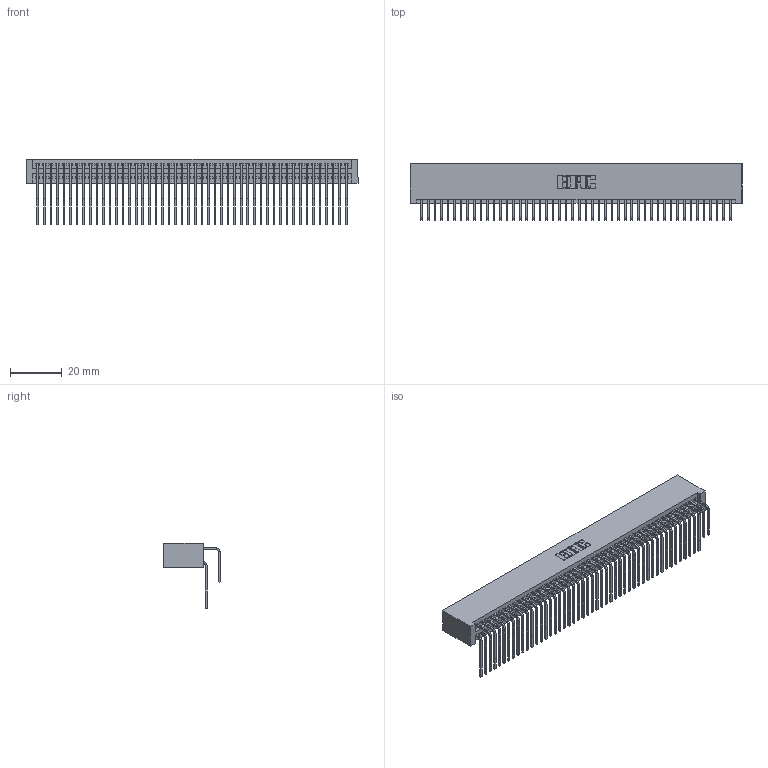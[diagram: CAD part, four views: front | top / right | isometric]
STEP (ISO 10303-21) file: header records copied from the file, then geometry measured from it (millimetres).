
FILE_DESCRIPTION (( 'STEP AP203' ), '1' );
FILE_NAME ('395-096-558-201.STEP', '2018-11-29T17:03:00', ( '' ), ( '' ), 'SwSTEP 2.0', 'SolidWorks 2016', '' );
FILE_SCHEMA (( 'CONFIG_CONTROL_DESIGN' ));
Length unit declared in the file: inch
Products named in the file (4): 345 Part_No Mounting Lugs; 345-292-001_558 559 Tail - 1; 345-292-001_558 Tail - 2; 395-096-558-201
Assembly tree (97 placements, depth 2):
  395-096-558-201
    345 Part_No Mounting Lugs
    345-292-001_558 559 Tail - 1  x48
    345-292-001_558 Tail - 2  x48
Bounding box: 128.52 x 21.83 x 25.53 mm (x, y, z)
Volume: 13710.4 mm3; surface area: 23289.8 mm2
Topology: 97 solids, 97 shells, 5110 faces, 15197 edges, 10002 vertices
Faces by surface type: plane 3436, cylinder 1674
Entity records: 38229 total; most frequent: CARTESIAN_POINT 6447, ORIENTED_EDGE 6330, DIRECTION 5645, EDGE_CURVE 3165, LINE 2809, VECTOR 2809, VERTEX_POINT 2106, AXIS2_PLACEMENT_3D 1418
